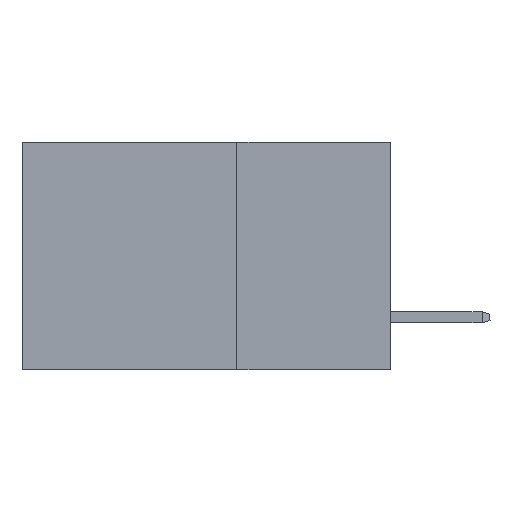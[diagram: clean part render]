
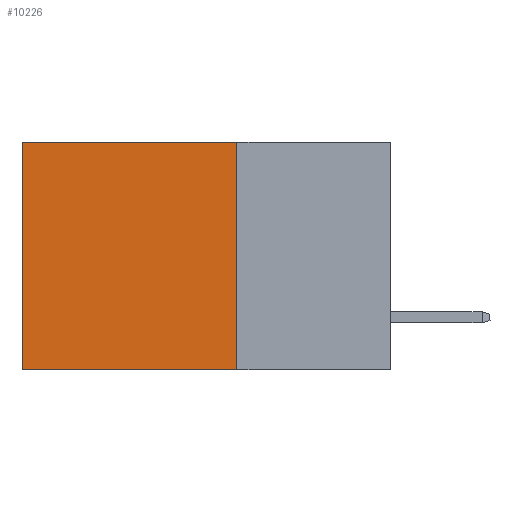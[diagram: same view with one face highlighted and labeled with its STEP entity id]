
A CAD part, left-side view. The second image highlights one B-rep face of the part: STEP entity #10226.
In plain terms, the highlighted planar face has unit normal (-1, 0, 0).
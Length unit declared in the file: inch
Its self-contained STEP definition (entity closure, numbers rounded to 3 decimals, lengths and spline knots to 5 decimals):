
#591 = CARTESIAN_POINT ( 'NONE',  ( 0.2875, 0.6, -0.37 ) ) ;
#894 = VECTOR ( 'NONE', #4152, 39.37008 ) ;
#1069 = VECTOR ( 'NONE', #8929, 39.37008 ) ;
#1075 = VERTEX_POINT ( 'NONE', #6614 ) ;
#1472 = LINE ( 'NONE', #7765, #1069 ) ;
#2410 = LINE ( 'NONE', #10802, #14190 ) ;
#2483 = CARTESIAN_POINT ( 'NONE',  ( 0.2875, 0.6, 0. ) ) ;
#2518 = EDGE_CURVE ( 'NONE', #11275, #9805, #2410, .T. ) ;
#2761 = VERTEX_POINT ( 'NONE', #2483 ) ;
#3597 = CARTESIAN_POINT ( 'NONE',  ( 0.2875, 0.25, -0.37 ) ) ;
#4152 = DIRECTION ( 'NONE',  ( 0., 0., -1. ) ) ;
#4304 = FACE_OUTER_BOUND ( 'NONE', #4790, .T. ) ;
#4790 = EDGE_LOOP ( 'NONE', ( #14089, #4943, #9087, #14142 ) ) ;
#4943 = ORIENTED_EDGE ( 'NONE', *, *, #2518, .F. ) ;
#6150 = CARTESIAN_POINT ( 'NONE',  ( 0.2875, 0.25, 0. ) ) ;
#6195 = DIRECTION ( 'NONE',  ( 1., 0., 0. ) ) ;
#6429 = CARTESIAN_POINT ( 'NONE',  ( 0.2875, 0.6, 0. ) ) ;
#6614 = CARTESIAN_POINT ( 'NONE',  ( 0.2875, 0.25, 0. ) ) ;
#6965 = CARTESIAN_POINT ( 'NONE',  ( 0.2875, 0.25, 0. ) ) ;
#7765 = CARTESIAN_POINT ( 'NONE',  ( 0.2875, 0.25, 0. ) ) ;
#8850 = VECTOR ( 'NONE', #11567, 39.37008 ) ;
#8929 = DIRECTION ( 'NONE',  ( 0., 0., -1. ) ) ;
#9087 = ORIENTED_EDGE ( 'NONE', *, *, #9796, .F. ) ;
#9174 = EDGE_CURVE ( 'NONE', #2761, #9805, #13600, .T. ) ;
#9796 = EDGE_CURVE ( 'NONE', #1075, #11275, #1472, .T. ) ;
#9805 = VERTEX_POINT ( 'NONE', #591 ) ;
#10226 = ADVANCED_FACE ( 'NONE', ( #4304 ), #13011, .F. ) ;
#10538 = EDGE_CURVE ( 'NONE', #1075, #2761, #11832, .T. ) ;
#10802 = CARTESIAN_POINT ( 'NONE',  ( 0.2875, 0.25, -0.37 ) ) ;
#11275 = VERTEX_POINT ( 'NONE', #3597 ) ;
#11567 = DIRECTION ( 'NONE',  ( 0., 1., 0. ) ) ;
#11654 = AXIS2_PLACEMENT_3D ( 'NONE', #6150, #6195, #14076 ) ;
#11832 = LINE ( 'NONE', #6965, #8850 ) ;
#13011 = PLANE ( 'NONE',  #11654 ) ;
#13600 = LINE ( 'NONE', #6429, #894 ) ;
#14076 = DIRECTION ( 'NONE',  ( 0., 0., -1. ) ) ;
#14089 = ORIENTED_EDGE ( 'NONE', *, *, #9174, .T. ) ;
#14142 = ORIENTED_EDGE ( 'NONE', *, *, #10538, .T. ) ;
#14190 = VECTOR ( 'NONE', #14206, 39.37008 ) ;
#14206 = DIRECTION ( 'NONE',  ( 0., 1., 0. ) ) ;
